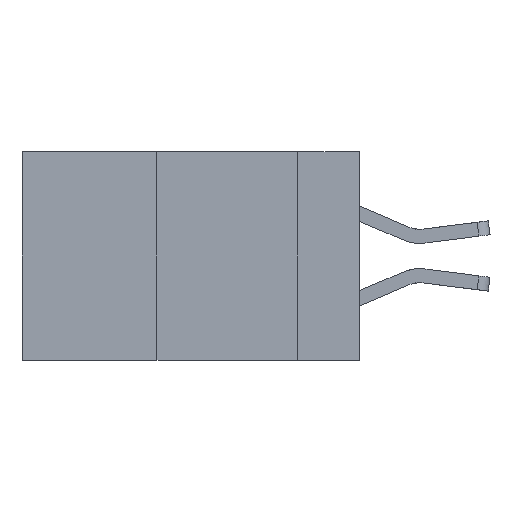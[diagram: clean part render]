
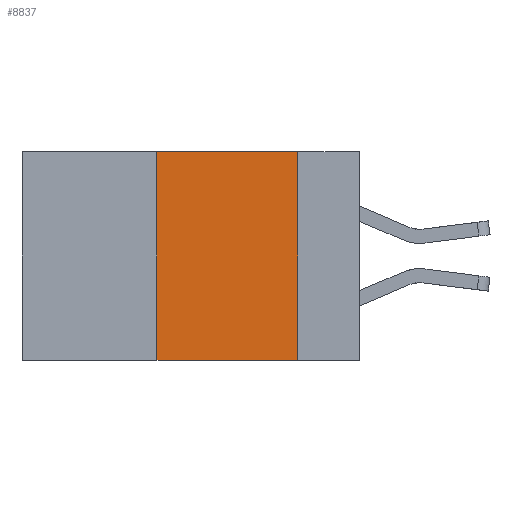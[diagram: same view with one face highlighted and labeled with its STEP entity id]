
A CAD part, left-side view. The second image highlights one B-rep face of the part: STEP entity #8837.
In plain terms, the highlighted planar face has unit normal (-1, 0, 0).
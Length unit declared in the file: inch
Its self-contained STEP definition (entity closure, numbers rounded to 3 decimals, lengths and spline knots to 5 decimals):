
#52 = CARTESIAN_POINT ( 'NONE',  ( 0., 0.11, 0. ) ) ;
#280 = LINE ( 'NONE', #10643, #9982 ) ;
#490 = CARTESIAN_POINT ( 'NONE',  ( 0., 0.6, -0.37 ) ) ;
#786 = AXIS2_PLACEMENT_3D ( 'NONE', #6288, #10803, #5385 ) ;
#906 = DIRECTION ( 'NONE',  ( 0., -1., 0. ) ) ;
#1182 = EDGE_CURVE ( 'NONE', #6978, #7161, #9367, .T. ) ;
#1233 = CARTESIAN_POINT ( 'NONE',  ( 0., 0.36, 0. ) ) ;
#1638 = CARTESIAN_POINT ( 'NONE',  ( 0., 0.11, -0.37 ) ) ;
#1675 = EDGE_LOOP ( 'NONE', ( #8143, #8264, #8701, #9430 ) ) ;
#2467 = PLANE ( 'NONE',  #786 ) ;
#3171 = EDGE_CURVE ( 'NONE', #6978, #5931, #280, .T. ) ;
#4610 = CARTESIAN_POINT ( 'NONE',  ( 0., 0.36, -0.37 ) ) ;
#5368 = VECTOR ( 'NONE', #10157, 39.37008 ) ;
#5385 = DIRECTION ( 'NONE',  ( 0., 0., -1. ) ) ;
#5931 = VERTEX_POINT ( 'NONE', #1233 ) ;
#6288 = CARTESIAN_POINT ( 'NONE',  ( 0., 0.6, 0. ) ) ;
#6392 = DIRECTION ( 'NONE',  ( 0., 0., 1. ) ) ;
#6615 = LINE ( 'NONE', #52, #11344 ) ;
#6781 = DIRECTION ( 'NONE',  ( 0., 0., -1. ) ) ;
#6978 = VERTEX_POINT ( 'NONE', #4610 ) ;
#7161 = VERTEX_POINT ( 'NONE', #1638 ) ;
#7703 = FACE_OUTER_BOUND ( 'NONE', #1675, .T. ) ;
#7708 = EDGE_CURVE ( 'NONE', #5931, #11244, #10216, .T. ) ;
#8143 = ORIENTED_EDGE ( 'NONE', *, *, #11418, .F. ) ;
#8264 = ORIENTED_EDGE ( 'NONE', *, *, #7708, .F. ) ;
#8701 = ORIENTED_EDGE ( 'NONE', *, *, #3171, .F. ) ;
#8837 = ADVANCED_FACE ( 'NONE', ( #7703 ), #2467, .F. ) ;
#9233 = CARTESIAN_POINT ( 'NONE',  ( 0., 0.11, 0. ) ) ;
#9367 = LINE ( 'NONE', #490, #10834 ) ;
#9430 = ORIENTED_EDGE ( 'NONE', *, *, #1182, .T. ) ;
#9982 = VECTOR ( 'NONE', #6392, 39.37008 ) ;
#10157 = DIRECTION ( 'NONE',  ( 0., -1., 0. ) ) ;
#10216 = LINE ( 'NONE', #10985, #5368 ) ;
#10643 = CARTESIAN_POINT ( 'NONE',  ( 0., 0.36, 0. ) ) ;
#10803 = DIRECTION ( 'NONE',  ( 1., 0., 0. ) ) ;
#10834 = VECTOR ( 'NONE', #906, 39.37008 ) ;
#10985 = CARTESIAN_POINT ( 'NONE',  ( 0., 0.6, 0. ) ) ;
#11244 = VERTEX_POINT ( 'NONE', #9233 ) ;
#11344 = VECTOR ( 'NONE', #6781, 39.37008 ) ;
#11418 = EDGE_CURVE ( 'NONE', #11244, #7161, #6615, .T. ) ;
